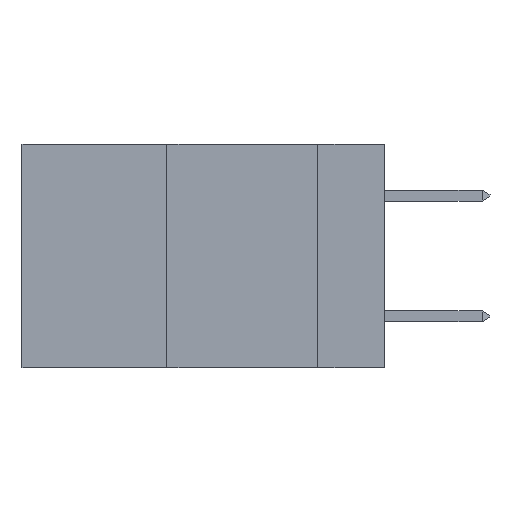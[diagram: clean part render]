
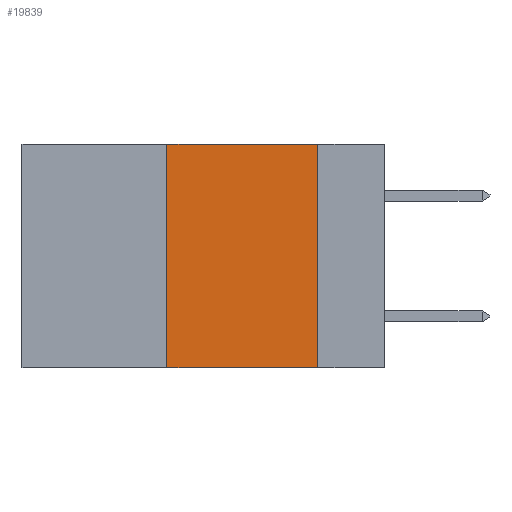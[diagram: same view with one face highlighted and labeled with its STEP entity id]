
A CAD part, left-side view. The second image highlights one B-rep face of the part: STEP entity #19839.
In plain terms, the highlighted planar face has unit normal (-1, 0, 0).
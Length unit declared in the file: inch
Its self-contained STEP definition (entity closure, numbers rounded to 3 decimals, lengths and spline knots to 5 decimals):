
#381 = CARTESIAN_POINT ( 'NONE',  ( 0., 0.11, 0. ) ) ;
#1157 = CARTESIAN_POINT ( 'NONE',  ( 0., 0.11, -0.37 ) ) ;
#1399 = CARTESIAN_POINT ( 'NONE',  ( 0., 0.11, 0. ) ) ;
#1438 = EDGE_CURVE ( 'NONE', #12917, #14099, #14877, .T. ) ;
#3275 = CARTESIAN_POINT ( 'NONE',  ( 0., 0.6, 0. ) ) ;
#3671 = CARTESIAN_POINT ( 'NONE',  ( 0., 0.6, -0.37 ) ) ;
#4268 = DIRECTION ( 'NONE',  ( 0., 0., 1. ) ) ;
#4536 = CARTESIAN_POINT ( 'NONE',  ( 0., 0.36, 0. ) ) ;
#6106 = ORIENTED_EDGE ( 'NONE', *, *, #16099, .F. ) ;
#7622 = ORIENTED_EDGE ( 'NONE', *, *, #1438, .F. ) ;
#8306 = AXIS2_PLACEMENT_3D ( 'NONE', #12824, #10853, #8642 ) ;
#8642 = DIRECTION ( 'NONE',  ( 0., 0., -1. ) ) ;
#9793 = CARTESIAN_POINT ( 'NONE',  ( 0., 0.36, 0. ) ) ;
#10627 = VERTEX_POINT ( 'NONE', #11091 ) ;
#10853 = DIRECTION ( 'NONE',  ( 1., 0., 0. ) ) ;
#11091 = CARTESIAN_POINT ( 'NONE',  ( 0., 0.36, -0.37 ) ) ;
#11710 = LINE ( 'NONE', #4536, #23689 ) ;
#12824 = CARTESIAN_POINT ( 'NONE',  ( 0., 0.6, 0. ) ) ;
#12917 = VERTEX_POINT ( 'NONE', #9793 ) ;
#13714 = LINE ( 'NONE', #3671, #13986 ) ;
#13986 = VECTOR ( 'NONE', #15490, 39.37008 ) ;
#14099 = VERTEX_POINT ( 'NONE', #381 ) ;
#14206 = LINE ( 'NONE', #1399, #18530 ) ;
#14258 = VECTOR ( 'NONE', #17562, 39.37008 ) ;
#14771 = VERTEX_POINT ( 'NONE', #1157 ) ;
#14877 = LINE ( 'NONE', #3275, #14258 ) ;
#15347 = FACE_OUTER_BOUND ( 'NONE', #17015, .T. ) ;
#15490 = DIRECTION ( 'NONE',  ( 0., -1., 0. ) ) ;
#15616 = DIRECTION ( 'NONE',  ( 0., 0., -1. ) ) ;
#16099 = EDGE_CURVE ( 'NONE', #10627, #12917, #11710, .T. ) ;
#17015 = EDGE_LOOP ( 'NONE', ( #21497, #7622, #6106, #19675 ) ) ;
#17562 = DIRECTION ( 'NONE',  ( 0., -1., 0. ) ) ;
#18317 = EDGE_CURVE ( 'NONE', #14099, #14771, #14206, .T. ) ;
#18530 = VECTOR ( 'NONE', #15616, 39.37008 ) ;
#19675 = ORIENTED_EDGE ( 'NONE', *, *, #22251, .T. ) ;
#19839 = ADVANCED_FACE ( 'NONE', ( #15347 ), #20709, .F. ) ;
#20709 = PLANE ( 'NONE',  #8306 ) ;
#21497 = ORIENTED_EDGE ( 'NONE', *, *, #18317, .F. ) ;
#22251 = EDGE_CURVE ( 'NONE', #10627, #14771, #13714, .T. ) ;
#23689 = VECTOR ( 'NONE', #4268, 39.37008 ) ;
